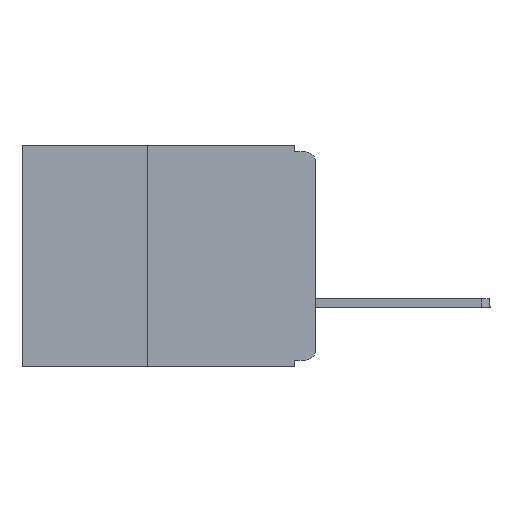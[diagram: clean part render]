
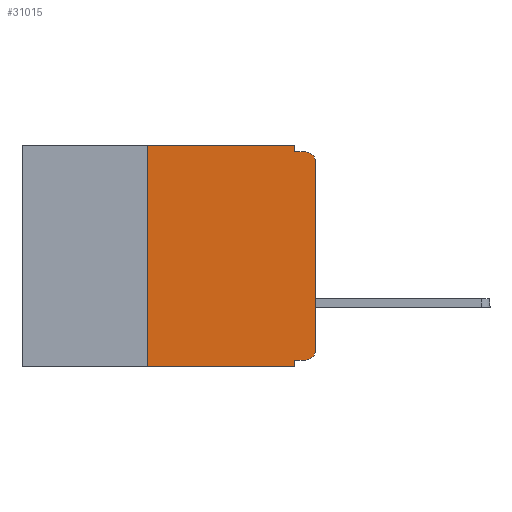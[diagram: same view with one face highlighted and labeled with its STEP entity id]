
A CAD part, left-side view. The second image highlights one B-rep face of the part: STEP entity #31015.
In plain terms, the highlighted planar face has unit normal (-1, 0, 0).
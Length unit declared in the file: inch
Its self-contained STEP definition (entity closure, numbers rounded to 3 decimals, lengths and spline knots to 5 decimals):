
#279 = DIRECTION ( 'NONE',  ( 0., 0., 1. ) ) ;
#1067 = AXIS2_PLACEMENT_3D ( 'NONE', #31759, #22026, #7123 ) ;
#1161 = CARTESIAN_POINT ( 'NONE',  ( 0., 0.031, -0.33 ) ) ;
#1868 = DIRECTION ( 'NONE',  ( 0., -1., 0. ) ) ;
#2513 = EDGE_CURVE ( 'NONE', #3032, #18161, #15925, .T. ) ;
#2896 = CARTESIAN_POINT ( 'NONE',  ( 0., 0., -0.025 ) ) ;
#3032 = VERTEX_POINT ( 'NONE', #8110 ) ;
#4040 = EDGE_CURVE ( 'NONE', #25077, #6158, #12641, .T. ) ;
#4266 = CARTESIAN_POINT ( 'NONE',  ( 0., 0., -0.01 ) ) ;
#5198 = VECTOR ( 'NONE', #19027, 39.37008 ) ;
#5491 = VECTOR ( 'NONE', #11375, 39.37008 ) ;
#5877 = ORIENTED_EDGE ( 'NONE', *, *, #27778, .T. ) ;
#6095 = EDGE_CURVE ( 'NONE', #25077, #17408, #16063, .T. ) ;
#6158 = VERTEX_POINT ( 'NONE', #7789 ) ;
#6259 = CARTESIAN_POINT ( 'NONE',  ( 0., 0.25, -0.33 ) ) ;
#6281 = LINE ( 'NONE', #8872, #5491 ) ;
#7123 = DIRECTION ( 'NONE',  ( 0., 0., -1. ) ) ;
#7392 = ORIENTED_EDGE ( 'NONE', *, *, #4040, .F. ) ;
#7789 = CARTESIAN_POINT ( 'NONE',  ( 0., 0.031, -0.32 ) ) ;
#8110 = CARTESIAN_POINT ( 'NONE',  ( 0., 0.031, 0. ) ) ;
#8316 = EDGE_CURVE ( 'NONE', #15177, #3032, #17470, .T. ) ;
#8872 = CARTESIAN_POINT ( 'NONE',  ( 0., 0.437, -0.33 ) ) ;
#9305 = VECTOR ( 'NONE', #24603, 39.37008 ) ;
#9630 = VECTOR ( 'NONE', #18811, 39.37008 ) ;
#9759 = DIRECTION ( 'NONE',  ( 0., 0., -1. ) ) ;
#9852 = DIRECTION ( 'NONE',  ( -1., 0., 0. ) ) ;
#9856 = CARTESIAN_POINT ( 'NONE',  ( 0., 0.015, -0.305 ) ) ;
#10249 = CARTESIAN_POINT ( 'NONE',  ( 0., 0., 0. ) ) ;
#10798 = VERTEX_POINT ( 'NONE', #2896 ) ;
#11031 = VERTEX_POINT ( 'NONE', #6259 ) ;
#11375 = DIRECTION ( 'NONE',  ( 0., -1., 0. ) ) ;
#11493 = CARTESIAN_POINT ( 'NONE',  ( 0., 0.25, -0.33 ) ) ;
#11535 = CARTESIAN_POINT ( 'NONE',  ( 0., 0.015, -0.32 ) ) ;
#11953 = CARTESIAN_POINT ( 'NONE',  ( 0., 0.437, 0. ) ) ;
#12617 = AXIS2_PLACEMENT_3D ( 'NONE', #13349, #30617, #15874 ) ;
#12641 = LINE ( 'NONE', #19100, #5198 ) ;
#13307 = CARTESIAN_POINT ( 'NONE',  ( 0., 0.25, 0. ) ) ;
#13349 = CARTESIAN_POINT ( 'NONE',  ( 0., 0.015, -0.025 ) ) ;
#13371 = CIRCLE ( 'NONE', #12617, 0.015 ) ;
#13495 = CARTESIAN_POINT ( 'NONE',  ( 0., 0.031, -0.01 ) ) ;
#14186 = VECTOR ( 'NONE', #279, 39.37008 ) ;
#14525 = AXIS2_PLACEMENT_3D ( 'NONE', #9856, #9852, #9759 ) ;
#15177 = VERTEX_POINT ( 'NONE', #13307 ) ;
#15733 = ORIENTED_EDGE ( 'NONE', *, *, #30373, .F. ) ;
#15874 = DIRECTION ( 'NONE',  ( 0., 0., -1. ) ) ;
#15925 = LINE ( 'NONE', #24246, #9305 ) ;
#16063 = CIRCLE ( 'NONE', #14525, 0.015 ) ;
#17408 = VERTEX_POINT ( 'NONE', #25715 ) ;
#17470 = LINE ( 'NONE', #11953, #27497 ) ;
#17657 = EDGE_CURVE ( 'NONE', #18161, #22092, #24444, .T. ) ;
#17877 = VECTOR ( 'NONE', #1868, 39.37008 ) ;
#18161 = VERTEX_POINT ( 'NONE', #13495 ) ;
#18163 = FACE_OUTER_BOUND ( 'NONE', #31104, .T. ) ;
#18811 = DIRECTION ( 'NONE',  ( 0., 0., 1. ) ) ;
#19027 = DIRECTION ( 'NONE',  ( 0., 1., 0. ) ) ;
#19100 = CARTESIAN_POINT ( 'NONE',  ( 0., 0., -0.32 ) ) ;
#19771 = VERTEX_POINT ( 'NONE', #1161 ) ;
#20035 = VECTOR ( 'NONE', #30110, 39.37008 ) ;
#20160 = EDGE_CURVE ( 'NONE', #17408, #10798, #20799, .T. ) ;
#20183 = EDGE_CURVE ( 'NONE', #6158, #19771, #21576, .T. ) ;
#20799 = LINE ( 'NONE', #10249, #14186 ) ;
#21576 = LINE ( 'NONE', #27668, #20035 ) ;
#21810 = PLANE ( 'NONE',  #1067 ) ;
#22026 = DIRECTION ( 'NONE',  ( 1., 0., 0. ) ) ;
#22092 = VERTEX_POINT ( 'NONE', #27266 ) ;
#24246 = CARTESIAN_POINT ( 'NONE',  ( 0., 0.031, 0. ) ) ;
#24444 = LINE ( 'NONE', #4266, #17877 ) ;
#24560 = DIRECTION ( 'NONE',  ( 0., -1., 0. ) ) ;
#24603 = DIRECTION ( 'NONE',  ( 0., 0., -1. ) ) ;
#25077 = VERTEX_POINT ( 'NONE', #11535 ) ;
#25260 = ORIENTED_EDGE ( 'NONE', *, *, #17657, .F. ) ;
#25715 = CARTESIAN_POINT ( 'NONE',  ( 0., 0., -0.305 ) ) ;
#26355 = ORIENTED_EDGE ( 'NONE', *, *, #6095, .T. ) ;
#26705 = ORIENTED_EDGE ( 'NONE', *, *, #2513, .F. ) ;
#27266 = CARTESIAN_POINT ( 'NONE',  ( 0., 0.015, -0.01 ) ) ;
#27497 = VECTOR ( 'NONE', #24560, 39.37008 ) ;
#27668 = CARTESIAN_POINT ( 'NONE',  ( 0., 0.031, -0.33 ) ) ;
#27778 = EDGE_CURVE ( 'NONE', #11031, #19771, #6281, .T. ) ;
#28094 = ORIENTED_EDGE ( 'NONE', *, *, #20160, .T. ) ;
#28590 = ORIENTED_EDGE ( 'NONE', *, *, #8316, .F. ) ;
#30110 = DIRECTION ( 'NONE',  ( 0., 0., -1. ) ) ;
#30124 = LINE ( 'NONE', #11493, #9630 ) ;
#30373 = EDGE_CURVE ( 'NONE', #11031, #15177, #30124, .T. ) ;
#30617 = DIRECTION ( 'NONE',  ( -1., 0., 0. ) ) ;
#30945 = ORIENTED_EDGE ( 'NONE', *, *, #20183, .F. ) ;
#31015 = ADVANCED_FACE ( 'NONE', ( #18163 ), #21810, .F. ) ;
#31104 = EDGE_LOOP ( 'NONE', ( #28094, #31280, #25260, #26705, #28590, #15733, #5877, #30945, #7392, #26355 ) ) ;
#31280 = ORIENTED_EDGE ( 'NONE', *, *, #31925, .T. ) ;
#31759 = CARTESIAN_POINT ( 'NONE',  ( 0., 0.437, 0. ) ) ;
#31925 = EDGE_CURVE ( 'NONE', #10798, #22092, #13371, .T. ) ;
